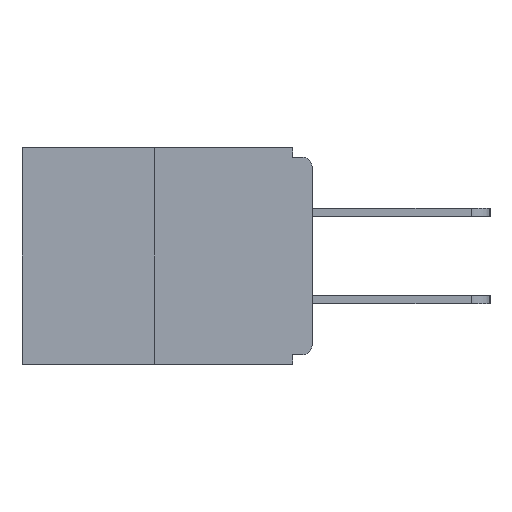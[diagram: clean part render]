
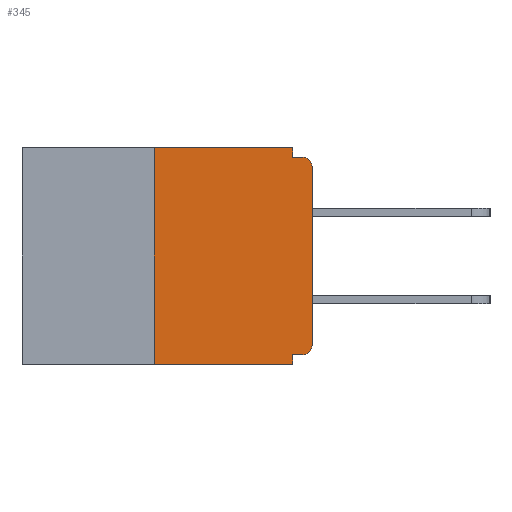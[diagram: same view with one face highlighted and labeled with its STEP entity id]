
A CAD part, left-side view. The second image highlights one B-rep face of the part: STEP entity #345.
In plain terms, the highlighted planar face has unit normal (-1, 0, 0).
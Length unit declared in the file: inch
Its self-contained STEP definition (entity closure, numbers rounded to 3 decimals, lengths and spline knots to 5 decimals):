
#7 = CARTESIAN_POINT ( 'NONE',  ( 0., 0.46, -0.343 ) ) ;
#25 = AXIS2_PLACEMENT_3D ( 'NONE', #6588, #15625, #15566 ) ;
#35 = VERTEX_POINT ( 'NONE', #13812 ) ;
#191 = VERTEX_POINT ( 'NONE', #8851 ) ;
#345 = ADVANCED_FACE ( 'NONE', ( #10514 ), #3749, .F. ) ;
#353 = EDGE_CURVE ( 'NONE', #7675, #4056, #11743, .T. ) ;
#1028 = ORIENTED_EDGE ( 'NONE', *, *, #16516, .F. ) ;
#1179 = VECTOR ( 'NONE', #6075, 39.37008 ) ;
#1220 = AXIS2_PLACEMENT_3D ( 'NONE', #6369, #16909, #7885 ) ;
#1358 = CARTESIAN_POINT ( 'NONE',  ( 0., 0.46, 0. ) ) ;
#1536 = VERTEX_POINT ( 'NONE', #1919 ) ;
#1544 = CARTESIAN_POINT ( 'NONE',  ( 0., 0.015, -0.03 ) ) ;
#1824 = ORIENTED_EDGE ( 'NONE', *, *, #4517, .F. ) ;
#1919 = CARTESIAN_POINT ( 'NONE',  ( 0., 0.031, -0.015 ) ) ;
#2103 = DIRECTION ( 'NONE',  ( 0., 0., -1. ) ) ;
#2470 = DIRECTION ( 'NONE',  ( 0., 1., 0. ) ) ;
#2493 = ORIENTED_EDGE ( 'NONE', *, *, #16224, .F. ) ;
#2763 = EDGE_CURVE ( 'NONE', #7675, #11439, #11684, .T. ) ;
#2801 = DIRECTION ( 'NONE',  ( 0., -1., 0. ) ) ;
#2876 = DIRECTION ( 'NONE',  ( -1., 0., 0. ) ) ;
#3006 = EDGE_CURVE ( 'NONE', #11439, #35, #7197, .T. ) ;
#3034 = CARTESIAN_POINT ( 'NONE',  ( 0., 0.031, -0.328 ) ) ;
#3044 = CARTESIAN_POINT ( 'NONE',  ( 0., 0.015, -0.328 ) ) ;
#3749 = PLANE ( 'NONE',  #25 ) ;
#4056 = VERTEX_POINT ( 'NONE', #15613 ) ;
#4517 = EDGE_CURVE ( 'NONE', #4963, #191, #5290, .T. ) ;
#4702 = DIRECTION ( 'NONE',  ( 0., 0., -1. ) ) ;
#4963 = VERTEX_POINT ( 'NONE', #16031 ) ;
#5290 = LINE ( 'NONE', #1358, #14664 ) ;
#5338 = DIRECTION ( 'NONE',  ( 0., -1., 0. ) ) ;
#5362 = VECTOR ( 'NONE', #2470, 39.37008 ) ;
#5598 = ORIENTED_EDGE ( 'NONE', *, *, #353, .T. ) ;
#6075 = DIRECTION ( 'NONE',  ( 0., 0., 1. ) ) ;
#6203 = CARTESIAN_POINT ( 'NONE',  ( 0., 0.25, 0. ) ) ;
#6359 = ORIENTED_EDGE ( 'NONE', *, *, #11064, .T. ) ;
#6369 = CARTESIAN_POINT ( 'NONE',  ( 0., 0.015, -0.313 ) ) ;
#6371 = CIRCLE ( 'NONE', #14967, 0.015 ) ;
#6576 = ORIENTED_EDGE ( 'NONE', *, *, #11318, .T. ) ;
#6588 = CARTESIAN_POINT ( 'NONE',  ( 0., 0.46, 0. ) ) ;
#6982 = LINE ( 'NONE', #14408, #12263 ) ;
#7177 = CARTESIAN_POINT ( 'NONE',  ( 0., 0.25, -0.343 ) ) ;
#7197 = LINE ( 'NONE', #8583, #15528 ) ;
#7419 = DIRECTION ( 'NONE',  ( 0., 0., 1. ) ) ;
#7610 = VECTOR ( 'NONE', #10590, 39.37008 ) ;
#7675 = VERTEX_POINT ( 'NONE', #3044 ) ;
#7885 = DIRECTION ( 'NONE',  ( 0., 0., -1. ) ) ;
#8160 = LINE ( 'NONE', #12375, #14060 ) ;
#8583 = CARTESIAN_POINT ( 'NONE',  ( 0., 0.031, -0.343 ) ) ;
#8851 = CARTESIAN_POINT ( 'NONE',  ( 0., 0.031, 0. ) ) ;
#9403 = CARTESIAN_POINT ( 'NONE',  ( 0., 0., -0.03 ) ) ;
#10514 = FACE_OUTER_BOUND ( 'NONE', #14089, .T. ) ;
#10554 = EDGE_CURVE ( 'NONE', #15904, #35, #11072, .T. ) ;
#10590 = DIRECTION ( 'NONE',  ( 0., -1., 0. ) ) ;
#10640 = DIRECTION ( 'NONE',  ( 0., 0., -1. ) ) ;
#10713 = ORIENTED_EDGE ( 'NONE', *, *, #2763, .F. ) ;
#11064 = EDGE_CURVE ( 'NONE', #4056, #11211, #6982, .T. ) ;
#11072 = LINE ( 'NONE', #7, #7610 ) ;
#11210 = VECTOR ( 'NONE', #5338, 39.37008 ) ;
#11211 = VERTEX_POINT ( 'NONE', #9403 ) ;
#11318 = EDGE_CURVE ( 'NONE', #11211, #15020, #6371, .T. ) ;
#11439 = VERTEX_POINT ( 'NONE', #3034 ) ;
#11684 = LINE ( 'NONE', #15413, #5362 ) ;
#11743 = CIRCLE ( 'NONE', #1220, 0.015 ) ;
#12263 = VECTOR ( 'NONE', #7419, 39.37008 ) ;
#12375 = CARTESIAN_POINT ( 'NONE',  ( 0., 0.031, 0. ) ) ;
#12647 = LINE ( 'NONE', #14439, #11210 ) ;
#12978 = LINE ( 'NONE', #6203, #1179 ) ;
#13380 = ORIENTED_EDGE ( 'NONE', *, *, #3006, .F. ) ;
#13573 = EDGE_CURVE ( 'NONE', #15904, #4963, #12978, .T. ) ;
#13812 = CARTESIAN_POINT ( 'NONE',  ( 0., 0.031, -0.343 ) ) ;
#14060 = VECTOR ( 'NONE', #2103, 39.37008 ) ;
#14089 = EDGE_LOOP ( 'NONE', ( #1824, #16147, #14745, #13380, #10713, #5598, #6359, #6576, #2493, #1028 ) ) ;
#14408 = CARTESIAN_POINT ( 'NONE',  ( 0., 0., 0. ) ) ;
#14439 = CARTESIAN_POINT ( 'NONE',  ( 0., 0., -0.015 ) ) ;
#14664 = VECTOR ( 'NONE', #2801, 39.37008 ) ;
#14745 = ORIENTED_EDGE ( 'NONE', *, *, #10554, .T. ) ;
#14967 = AXIS2_PLACEMENT_3D ( 'NONE', #1544, #2876, #10640 ) ;
#15020 = VERTEX_POINT ( 'NONE', #16038 ) ;
#15413 = CARTESIAN_POINT ( 'NONE',  ( 0., 0., -0.328 ) ) ;
#15528 = VECTOR ( 'NONE', #4702, 39.37008 ) ;
#15566 = DIRECTION ( 'NONE',  ( 0., 0., -1. ) ) ;
#15613 = CARTESIAN_POINT ( 'NONE',  ( 0., 0., -0.313 ) ) ;
#15625 = DIRECTION ( 'NONE',  ( 1., 0., 0. ) ) ;
#15904 = VERTEX_POINT ( 'NONE', #7177 ) ;
#16031 = CARTESIAN_POINT ( 'NONE',  ( 0., 0.25, 0. ) ) ;
#16038 = CARTESIAN_POINT ( 'NONE',  ( 0., 0.015, -0.015 ) ) ;
#16147 = ORIENTED_EDGE ( 'NONE', *, *, #13573, .F. ) ;
#16224 = EDGE_CURVE ( 'NONE', #1536, #15020, #12647, .T. ) ;
#16516 = EDGE_CURVE ( 'NONE', #191, #1536, #8160, .T. ) ;
#16909 = DIRECTION ( 'NONE',  ( -1., 0., 0. ) ) ;
